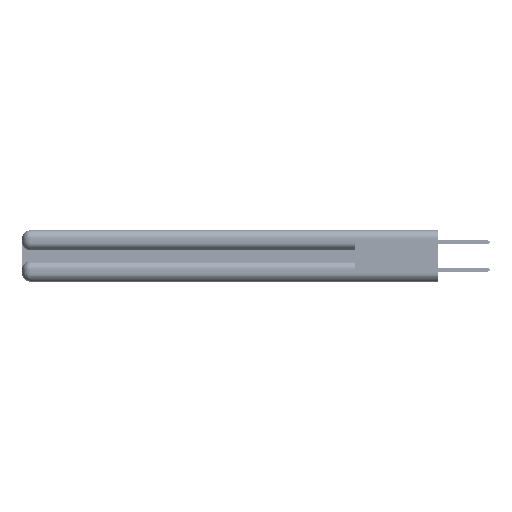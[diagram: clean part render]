
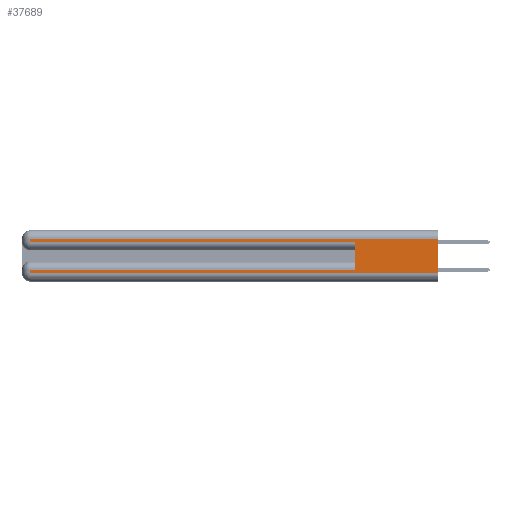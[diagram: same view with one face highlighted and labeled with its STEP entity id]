
A CAD part, left-side view. The second image highlights one B-rep face of the part: STEP entity #37689.
In plain terms, the highlighted planar face has unit normal (-1, 0, 0).
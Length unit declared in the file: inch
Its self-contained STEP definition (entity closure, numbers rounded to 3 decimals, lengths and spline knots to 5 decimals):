
#1545 = CARTESIAN_POINT ( 'NONE',  ( 0., 0., 0.06 ) ) ;
#1832 = EDGE_LOOP ( 'NONE', ( #19357, #13438, #37515, #32225, #21579, #7685, #46140, #31776 ) ) ;
#2099 = DIRECTION ( 'NONE',  ( 0., -1., 0. ) ) ;
#3248 = LINE ( 'NONE', #15976, #9189 ) ;
#4162 = CARTESIAN_POINT ( 'NONE',  ( 0., 0., 0.37 ) ) ;
#4397 = VERTEX_POINT ( 'NONE', #19722 ) ;
#5575 = VECTOR ( 'NONE', #17954, 39.37008 ) ;
#7172 = DIRECTION ( 'NONE',  ( 0., 0., 1. ) ) ;
#7685 = ORIENTED_EDGE ( 'NONE', *, *, #22136, .T. ) ;
#7858 = CARTESIAN_POINT ( 'NONE',  ( 0., 0., 0.31 ) ) ;
#8216 = CARTESIAN_POINT ( 'NONE',  ( 0., 0., 0.085 ) ) ;
#8769 = PLANE ( 'NONE',  #12250 ) ;
#9189 = VECTOR ( 'NONE', #32856, 39.37008 ) ;
#9992 = EDGE_CURVE ( 'NONE', #36046, #19758, #16469, .T. ) ;
#11279 = CARTESIAN_POINT ( 'NONE',  ( 0., 0., 0.37 ) ) ;
#12250 = AXIS2_PLACEMENT_3D ( 'NONE', #4162, #33557, #25292 ) ;
#12902 = VECTOR ( 'NONE', #37582, 39.37008 ) ;
#13438 = ORIENTED_EDGE ( 'NONE', *, *, #9992, .T. ) ;
#14051 = VERTEX_POINT ( 'NONE', #36846 ) ;
#14420 = CARTESIAN_POINT ( 'NONE',  ( 0., 2.94, 0.06 ) ) ;
#15898 = CARTESIAN_POINT ( 'NONE',  ( 0., 0., 0.06 ) ) ;
#15976 = CARTESIAN_POINT ( 'NONE',  ( 0., 2.94, 0.37 ) ) ;
#16469 = LINE ( 'NONE', #7858, #53290 ) ;
#16817 = CARTESIAN_POINT ( 'NONE',  ( 0., 2.94, 0.37 ) ) ;
#17954 = DIRECTION ( 'NONE',  ( 0., -1., 0. ) ) ;
#19357 = ORIENTED_EDGE ( 'NONE', *, *, #41648, .F. ) ;
#19722 = CARTESIAN_POINT ( 'NONE',  ( 0., 0.6, 0.285 ) ) ;
#19758 = VERTEX_POINT ( 'NONE', #52446 ) ;
#20586 = CARTESIAN_POINT ( 'NONE',  ( 0., 0.6, 0.145 ) ) ;
#21579 = ORIENTED_EDGE ( 'NONE', *, *, #25496, .F. ) ;
#22092 = VERTEX_POINT ( 'NONE', #24551 ) ;
#22136 = EDGE_CURVE ( 'NONE', #14051, #22092, #26702, .T. ) ;
#23955 = DIRECTION ( 'NONE',  ( 0., 0., -1. ) ) ;
#24399 = VECTOR ( 'NONE', #2099, 39.37008 ) ;
#24551 = CARTESIAN_POINT ( 'NONE',  ( 0., 2.94, 0.085 ) ) ;
#25292 = DIRECTION ( 'NONE',  ( 0., 0., -1. ) ) ;
#25496 = EDGE_CURVE ( 'NONE', #14051, #4397, #32776, .T. ) ;
#26702 = LINE ( 'NONE', #8216, #12902 ) ;
#28366 = LINE ( 'NONE', #1545, #24399 ) ;
#28849 = VERTEX_POINT ( 'NONE', #15898 ) ;
#31556 = CARTESIAN_POINT ( 'NONE',  ( 0., 2.94, 0.285 ) ) ;
#31683 = EDGE_CURVE ( 'NONE', #19758, #49629, #49764, .T. ) ;
#31776 = ORIENTED_EDGE ( 'NONE', *, *, #52600, .T. ) ;
#32225 = ORIENTED_EDGE ( 'NONE', *, *, #47145, .T. ) ;
#32776 = LINE ( 'NONE', #20586, #41954 ) ;
#32856 = DIRECTION ( 'NONE',  ( 0., 0., -1. ) ) ;
#33557 = DIRECTION ( 'NONE',  ( 1., 0., 0. ) ) ;
#35228 = CARTESIAN_POINT ( 'NONE',  ( 0., 0., 0.31 ) ) ;
#36046 = VERTEX_POINT ( 'NONE', #35228 ) ;
#36846 = CARTESIAN_POINT ( 'NONE',  ( 0., 0.6, 0.085 ) ) ;
#37515 = ORIENTED_EDGE ( 'NONE', *, *, #31683, .T. ) ;
#37548 = EDGE_CURVE ( 'NONE', #22092, #47694, #3248, .T. ) ;
#37582 = DIRECTION ( 'NONE',  ( 0., 1., 0. ) ) ;
#37689 = ADVANCED_FACE ( 'NONE', ( #42668 ), #8769, .F. ) ;
#41620 = DIRECTION ( 'NONE',  ( 0., 1., 0. ) ) ;
#41627 = LINE ( 'NONE', #11279, #46222 ) ;
#41648 = EDGE_CURVE ( 'NONE', #36046, #28849, #41627, .T. ) ;
#41954 = VECTOR ( 'NONE', #7172, 39.37008 ) ;
#42668 = FACE_OUTER_BOUND ( 'NONE', #1832, .T. ) ;
#46140 = ORIENTED_EDGE ( 'NONE', *, *, #37548, .T. ) ;
#46222 = VECTOR ( 'NONE', #23955, 39.37008 ) ;
#46520 = DIRECTION ( 'NONE',  ( 0., 0., -1. ) ) ;
#47145 = EDGE_CURVE ( 'NONE', #49629, #4397, #48254, .T. ) ;
#47694 = VERTEX_POINT ( 'NONE', #14420 ) ;
#47855 = CARTESIAN_POINT ( 'NONE',  ( 0., 0., 0.285 ) ) ;
#48254 = LINE ( 'NONE', #47855, #5575 ) ;
#49629 = VERTEX_POINT ( 'NONE', #31556 ) ;
#49764 = LINE ( 'NONE', #16817, #53724 ) ;
#52446 = CARTESIAN_POINT ( 'NONE',  ( 0., 2.94, 0.31 ) ) ;
#52600 = EDGE_CURVE ( 'NONE', #47694, #28849, #28366, .T. ) ;
#53290 = VECTOR ( 'NONE', #41620, 39.37008 ) ;
#53724 = VECTOR ( 'NONE', #46520, 39.37008 ) ;
